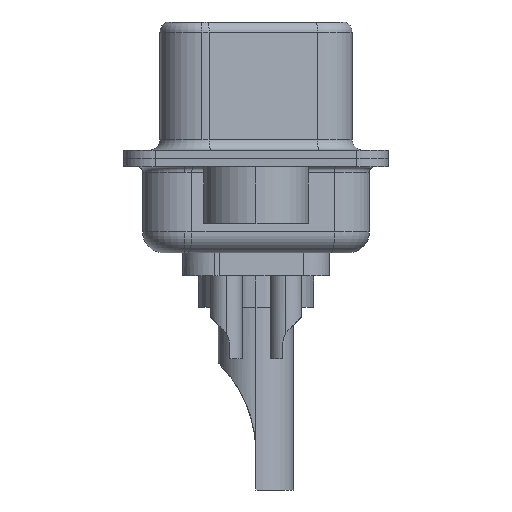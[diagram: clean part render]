
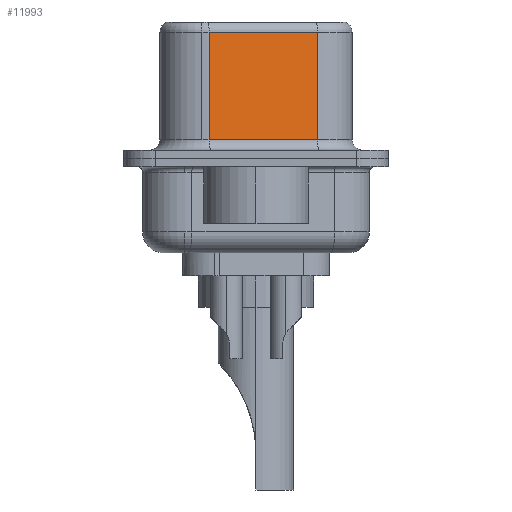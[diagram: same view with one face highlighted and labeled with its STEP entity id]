
A CAD part, left-side view. The second image highlights one B-rep face of the part: STEP entity #11993.
In plain terms, the highlighted planar face has unit normal (-0.985, -0.174, 0).
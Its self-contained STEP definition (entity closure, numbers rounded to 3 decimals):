
#1965 = ORIENTED_EDGE ( 'NONE', *, *, #5584, .T. ) ;
#2813 = LINE ( 'NONE', #13991, #18914 ) ;
#3116 = CARTESIAN_POINT ( 'NONE',  ( 4.565, -2.927, 6.52 ) ) ;
#4046 = EDGE_LOOP ( 'NONE', ( #8420, #20150, #9808, #1965 ) ) ;
#5081 = CARTESIAN_POINT ( 'NONE',  ( 4.565, -2.927, 6.52 ) ) ;
#5129 = EDGE_CURVE ( 'NONE', #16345, #13959, #2813, .T. ) ;
#5202 = LINE ( 'NONE', #16942, #13998 ) ;
#5584 = EDGE_CURVE ( 'NONE', #9623, #16179, #5202, .T. ) ;
#5749 = AXIS2_PLACEMENT_3D ( 'NONE', #5081, #8189, #19176 ) ;
#5756 = FACE_OUTER_BOUND ( 'NONE', #4046, .T. ) ;
#6312 = LINE ( 'NONE', #3116, #18284 ) ;
#6318 = VECTOR ( 'NONE', #15042, 1000. ) ;
#7777 = DIRECTION ( 'NONE',  ( 0., 0., -1. ) ) ;
#8189 = DIRECTION ( 'NONE',  ( 0.985, 0.174, 0. ) ) ;
#8420 = ORIENTED_EDGE ( 'NONE', *, *, #8681, .F. ) ;
#8576 = CARTESIAN_POINT ( 'NONE',  ( 4.565, -2.927, 0.9 ) ) ;
#8681 = EDGE_CURVE ( 'NONE', #16345, #16179, #6312, .T. ) ;
#9356 = CARTESIAN_POINT ( 'NONE',  ( 3.655, 2.233, 6.02 ) ) ;
#9623 = VERTEX_POINT ( 'NONE', #15292 ) ;
#9808 = ORIENTED_EDGE ( 'NONE', *, *, #19511, .T. ) ;
#10293 = CARTESIAN_POINT ( 'NONE',  ( 3.655, 2.233, 6.52 ) ) ;
#10448 = LINE ( 'NONE', #10293, #6318 ) ;
#11993 = ADVANCED_FACE ( 'NONE', ( #5756 ), #12856, .F. ) ;
#12014 = DIRECTION ( 'NONE',  ( -0.174, 0.985, 0. ) ) ;
#12856 = PLANE ( 'NONE',  #5749 ) ;
#13959 = VERTEX_POINT ( 'NONE', #9356 ) ;
#13991 = CARTESIAN_POINT ( 'NONE',  ( 4.565, -2.927, 6.02 ) ) ;
#13998 = VECTOR ( 'NONE', #16945, 1000. ) ;
#15042 = DIRECTION ( 'NONE',  ( 0., 0., -1. ) ) ;
#15292 = CARTESIAN_POINT ( 'NONE',  ( 3.655, 2.233, 0.9 ) ) ;
#16179 = VERTEX_POINT ( 'NONE', #8576 ) ;
#16345 = VERTEX_POINT ( 'NONE', #16827 ) ;
#16827 = CARTESIAN_POINT ( 'NONE',  ( 4.565, -2.927, 6.02 ) ) ;
#16942 = CARTESIAN_POINT ( 'NONE',  ( 4.565, -2.927, 0.9 ) ) ;
#16945 = DIRECTION ( 'NONE',  ( 0.174, -0.985, 0. ) ) ;
#18284 = VECTOR ( 'NONE', #7777, 1000. ) ;
#18914 = VECTOR ( 'NONE', #12014, 1000. ) ;
#19176 = DIRECTION ( 'NONE',  ( -0.174, 0.985, 0. ) ) ;
#19511 = EDGE_CURVE ( 'NONE', #13959, #9623, #10448, .T. ) ;
#20150 = ORIENTED_EDGE ( 'NONE', *, *, #5129, .T. ) ;
